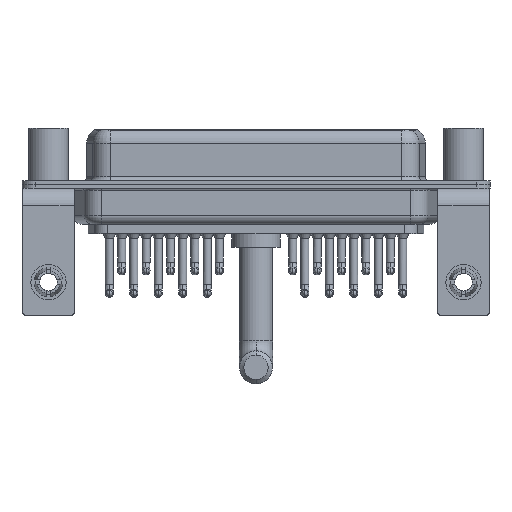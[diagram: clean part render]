
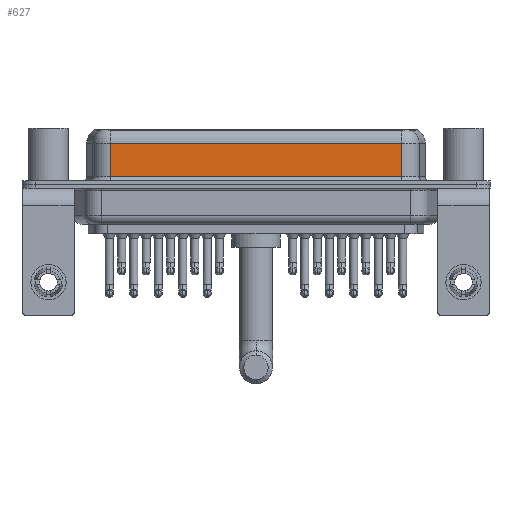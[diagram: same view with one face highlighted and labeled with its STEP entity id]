
A CAD part, front view. The second image highlights one B-rep face of the part: STEP entity #627.
In plain terms, the highlighted planar face has unit normal (0, -1, 0).
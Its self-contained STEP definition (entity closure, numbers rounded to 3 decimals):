
#627 = ADVANCED_FACE ( 'NONE', ( #12213 ), #5582, .F. ) ;
#815 = CARTESIAN_POINT ( 'NONE',  ( 7.013, -3.95, 4.65 ) ) ;
#2254 = LINE ( 'NONE', #20805, #9908 ) ;
#2728 = LINE ( 'NONE', #22911, #3241 ) ;
#2955 = CARTESIAN_POINT ( 'NONE',  ( 40.037, -3.95, 4.65 ) ) ;
#3241 = VECTOR ( 'NONE', #12757, 1000. ) ;
#3907 = CARTESIAN_POINT ( 'NONE',  ( 40.037, -3.95, 6.4 ) ) ;
#4078 = EDGE_CURVE ( 'NONE', #21588, #14264, #2728, .T. ) ;
#4789 = VERTEX_POINT ( 'NONE', #24041 ) ;
#5560 = EDGE_CURVE ( 'NONE', #14264, #20124, #2254, .T. ) ;
#5582 = PLANE ( 'NONE',  #5768 ) ;
#5768 = AXIS2_PLACEMENT_3D ( 'NONE', #14098, #7903, #18182 ) ;
#6952 = ORIENTED_EDGE ( 'NONE', *, *, #19188, .T. ) ;
#7903 = DIRECTION ( 'NONE',  ( 0., 1., 0. ) ) ;
#8205 = EDGE_CURVE ( 'NONE', #4789, #20124, #17972, .T. ) ;
#8878 = ORIENTED_EDGE ( 'NONE', *, *, #5560, .T. ) ;
#9427 = ORIENTED_EDGE ( 'NONE', *, *, #4078, .T. ) ;
#9908 = VECTOR ( 'NONE', #14832, 1000. ) ;
#10442 = ORIENTED_EDGE ( 'NONE', *, *, #8205, .F. ) ;
#12164 = DIRECTION ( 'NONE',  ( 0., 0., -1. ) ) ;
#12213 = FACE_OUTER_BOUND ( 'NONE', #18832, .T. ) ;
#12757 = DIRECTION ( 'NONE',  ( 0., 0., -1. ) ) ;
#13901 = VECTOR ( 'NONE', #12164, 1000. ) ;
#14089 = CARTESIAN_POINT ( 'NONE',  ( 7.013, -3.95, 0.9 ) ) ;
#14098 = CARTESIAN_POINT ( 'NONE',  ( 40.037, -3.95, 6.4 ) ) ;
#14264 = VERTEX_POINT ( 'NONE', #14089 ) ;
#14832 = DIRECTION ( 'NONE',  ( 1., 0., 0. ) ) ;
#15534 = DIRECTION ( 'NONE',  ( -1., 0., 0. ) ) ;
#17972 = LINE ( 'NONE', #3907, #13901 ) ;
#18182 = DIRECTION ( 'NONE',  ( 0., 0., 1. ) ) ;
#18683 = CARTESIAN_POINT ( 'NONE',  ( 40.037, -3.95, 0.9 ) ) ;
#18832 = EDGE_LOOP ( 'NONE', ( #10442, #6952, #9427, #8878 ) ) ;
#19106 = VECTOR ( 'NONE', #15534, 1000. ) ;
#19188 = EDGE_CURVE ( 'NONE', #4789, #21588, #23804, .T. ) ;
#20124 = VERTEX_POINT ( 'NONE', #18683 ) ;
#20805 = CARTESIAN_POINT ( 'NONE',  ( 40.037, -3.95, 0.9 ) ) ;
#21588 = VERTEX_POINT ( 'NONE', #815 ) ;
#22911 = CARTESIAN_POINT ( 'NONE',  ( 7.013, -3.95, 6.4 ) ) ;
#23804 = LINE ( 'NONE', #2955, #19106 ) ;
#24041 = CARTESIAN_POINT ( 'NONE',  ( 40.037, -3.95, 4.65 ) ) ;
